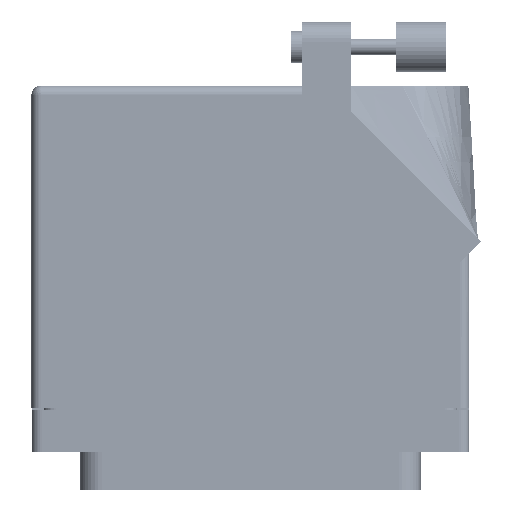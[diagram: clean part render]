
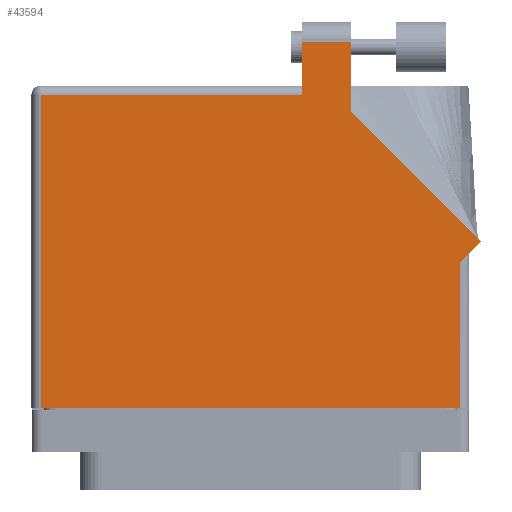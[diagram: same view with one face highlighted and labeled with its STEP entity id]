
A CAD part, front view. The second image highlights one B-rep face of the part: STEP entity #43594.
In plain terms, the highlighted face is planar.
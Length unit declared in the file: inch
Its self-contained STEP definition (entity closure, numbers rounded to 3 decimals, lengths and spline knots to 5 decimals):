
#3713 = CARTESIAN_POINT ( 'NONE',  ( 1.3155, 0.818, 0.765 ) ) ;
#3757 = VERTEX_POINT ( 'NONE', #68132 ) ;
#3786 = VERTEX_POINT ( 'NONE', #38550 ) ;
#4070 = VECTOR ( 'NONE', #32786, 39.37008 ) ;
#5472 = VERTEX_POINT ( 'NONE', #76003 ) ;
#6160 = DIRECTION ( 'NONE',  ( -1., 0., 0. ) ) ;
#7107 = VERTEX_POINT ( 'NONE', #30711 ) ;
#7168 = CARTESIAN_POINT ( 'NONE',  ( -1.3155, -0.1, 0.765 ) ) ;
#7425 = ORIENTED_EDGE ( 'NONE', *, *, #69309, .T. ) ;
#7524 = DIRECTION ( 'NONE',  ( -0.707, 0.707, 0. ) ) ;
#10588 = CARTESIAN_POINT ( 'NONE',  ( 1.44821, 0.95071, 0.765 ) ) ;
#12609 = VERTEX_POINT ( 'NONE', #83929 ) ;
#15305 = FACE_OUTER_BOUND ( 'NONE', #62200, .T. ) ;
#15928 = CARTESIAN_POINT ( 'NONE',  ( 1.44821, 0.95071, 0.765 ) ) ;
#16052 = DIRECTION ( 'NONE',  ( 1., 0., 0. ) ) ;
#17216 = LINE ( 'NONE', #51419, #20412 ) ;
#18614 = DIRECTION ( 'NONE',  ( -1., 0., 0. ) ) ;
#20081 = CARTESIAN_POINT ( 'NONE',  ( 0.3275, 1.93, 0.765 ) ) ;
#20128 = LINE ( 'NONE', #20081, #85169 ) ;
#20412 = VECTOR ( 'NONE', #16052, 39.37008 ) ;
#22193 = CARTESIAN_POINT ( 'NONE',  ( 1.3775, 0.88, 0.765 ) ) ;
#23041 = ORIENTED_EDGE ( 'NONE', *, *, #53617, .T. ) ;
#23342 = ORIENTED_EDGE ( 'NONE', *, *, #83880, .T. ) ;
#24243 = LINE ( 'NONE', #90247, #46632 ) ;
#24329 = VECTOR ( 'NONE', #18614, 39.37008 ) ;
#28575 = LINE ( 'NONE', #39365, #4070 ) ;
#29049 = DIRECTION ( 'NONE',  ( 0., 0., -1. ) ) ;
#30711 = CARTESIAN_POINT ( 'NONE',  ( -1.3155, 1.868, 0.765 ) ) ;
#32108 = VECTOR ( 'NONE', #73512, 39.37008 ) ;
#32587 = ORIENTED_EDGE ( 'NONE', *, *, #32824, .T. ) ;
#32786 = DIRECTION ( 'NONE',  ( 0., 1., 0. ) ) ;
#32824 = EDGE_CURVE ( 'NONE', #5472, #70871, #28575, .T. ) ;
#35370 = VECTOR ( 'NONE', #6160, 39.37008 ) ;
#38550 = CARTESIAN_POINT ( 'NONE',  ( 0.3275, 1.868, 0.765 ) ) ;
#39365 = CARTESIAN_POINT ( 'NONE',  ( 1.3155, 0.88, 0.765 ) ) ;
#41278 = ORIENTED_EDGE ( 'NONE', *, *, #63665, .T. ) ;
#41796 = VERTEX_POINT ( 'NONE', #7168 ) ;
#43463 = LINE ( 'NONE', #73856, #24329 ) ;
#43594 = ADVANCED_FACE ( 'NONE', ( #15305 ), #70219, .F. ) ;
#44722 = AXIS2_PLACEMENT_3D ( 'NONE', #71768, #29049, #72386 ) ;
#46632 = VECTOR ( 'NONE', #91473, 39.37008 ) ;
#46969 = VECTOR ( 'NONE', #7524, 39.37008 ) ;
#46985 = EDGE_CURVE ( 'NONE', #7107, #41796, #74838, .T. ) ;
#48893 = DIRECTION ( 'NONE',  ( 0., -1., 0. ) ) ;
#51375 = VECTOR ( 'NONE', #79606, 39.37008 ) ;
#51419 = CARTESIAN_POINT ( 'NONE',  ( -1.3775, -0.1, 0.765 ) ) ;
#53617 = EDGE_CURVE ( 'NONE', #74903, #3757, #66138, .T. ) ;
#54481 = LINE ( 'NONE', #83851, #35370 ) ;
#56053 = EDGE_CURVE ( 'NONE', #3757, #12609, #24243, .T. ) ;
#61958 = CARTESIAN_POINT ( 'NONE',  ( 0.3275, 2.205, 0.765 ) ) ;
#62200 = EDGE_LOOP ( 'NONE', ( #70164, #7425, #76149, #41278, #71188, #23342, #32587, #90366, #23041 ) ) ;
#63665 = EDGE_CURVE ( 'NONE', #3786, #7107, #54481, .T. ) ;
#66138 = LINE ( 'NONE', #15928, #46969 ) ;
#68132 = CARTESIAN_POINT ( 'NONE',  ( 0.6345, 1.76442, 0.765 ) ) ;
#68539 = EDGE_CURVE ( 'NONE', #70871, #74903, #78346, .T. ) ;
#68884 = VERTEX_POINT ( 'NONE', #61958 ) ;
#69309 = EDGE_CURVE ( 'NONE', #12609, #68884, #43463, .T. ) ;
#70164 = ORIENTED_EDGE ( 'NONE', *, *, #56053, .T. ) ;
#70219 = PLANE ( 'NONE',  #44722 ) ;
#70871 = VERTEX_POINT ( 'NONE', #3713 ) ;
#71188 = ORIENTED_EDGE ( 'NONE', *, *, #46985, .T. ) ;
#71768 = CARTESIAN_POINT ( 'NONE',  ( -1.3775, 1.93, 0.765 ) ) ;
#72386 = DIRECTION ( 'NONE',  ( -1., 0., 0. ) ) ;
#73512 = DIRECTION ( 'NONE',  ( 0., -1., 0. ) ) ;
#73856 = CARTESIAN_POINT ( 'NONE',  ( 0.3275, 2.205, 0.765 ) ) ;
#74838 = LINE ( 'NONE', #79777, #32108 ) ;
#74903 = VERTEX_POINT ( 'NONE', #10588 ) ;
#76003 = CARTESIAN_POINT ( 'NONE',  ( 1.3155, -0.1, 0.765 ) ) ;
#76149 = ORIENTED_EDGE ( 'NONE', *, *, #79844, .T. ) ;
#78346 = LINE ( 'NONE', #22193, #51375 ) ;
#79606 = DIRECTION ( 'NONE',  ( 0.707, 0.707, 0. ) ) ;
#79777 = CARTESIAN_POINT ( 'NONE',  ( -1.3155, -0.1, 0.765 ) ) ;
#79844 = EDGE_CURVE ( 'NONE', #68884, #3786, #20128, .T. ) ;
#83851 = CARTESIAN_POINT ( 'NONE',  ( -1.3775, 1.868, 0.765 ) ) ;
#83880 = EDGE_CURVE ( 'NONE', #41796, #5472, #17216, .T. ) ;
#83929 = CARTESIAN_POINT ( 'NONE',  ( 0.6345, 2.205, 0.765 ) ) ;
#85169 = VECTOR ( 'NONE', #48893, 39.37008 ) ;
#90247 = CARTESIAN_POINT ( 'NONE',  ( 0.6345, 1.76442, 0.765 ) ) ;
#90366 = ORIENTED_EDGE ( 'NONE', *, *, #68539, .T. ) ;
#91473 = DIRECTION ( 'NONE',  ( 0., 1., 0. ) ) ;
